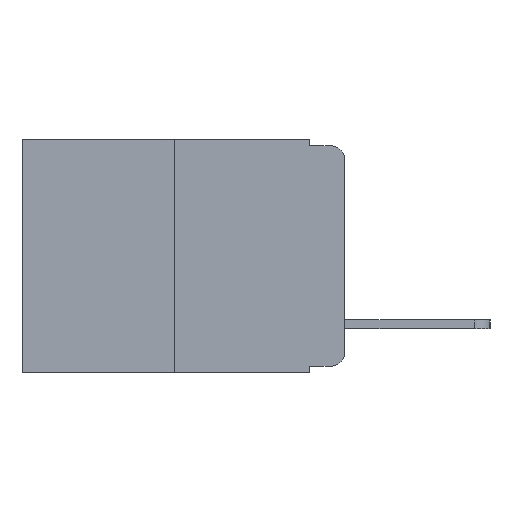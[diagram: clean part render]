
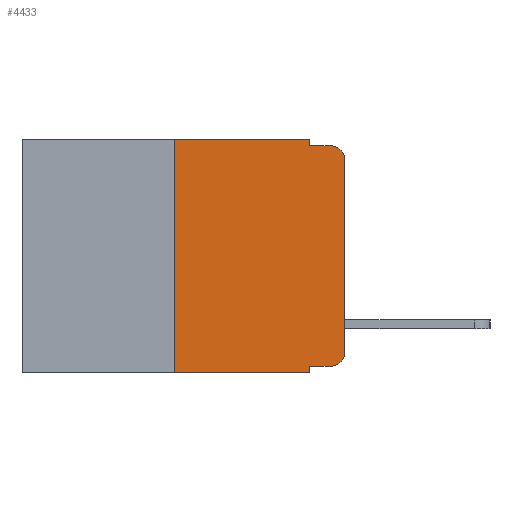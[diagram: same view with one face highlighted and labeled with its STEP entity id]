
A CAD part, left-side view. The second image highlights one B-rep face of the part: STEP entity #4433.
In plain terms, the highlighted planar face has unit normal (-1, 0, 0).
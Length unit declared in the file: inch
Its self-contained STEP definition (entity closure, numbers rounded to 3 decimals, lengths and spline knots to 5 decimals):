
#438 = ORIENTED_EDGE ( 'NONE', *, *, #14048, .F. ) ;
#652 = DIRECTION ( 'NONE',  ( -1., 0., 0. ) ) ;
#881 = EDGE_LOOP ( 'NONE', ( #9283, #4237, #18807, #438, #3809, #8578, #16939, #17595, #15039, #2555 ) ) ;
#1062 = CARTESIAN_POINT ( 'NONE',  ( 0., 0.473, -0.343 ) ) ;
#1090 = CARTESIAN_POINT ( 'NONE',  ( 0., 0.051, -0.01 ) ) ;
#1102 = VERTEX_POINT ( 'NONE', #14629 ) ;
#1168 = CARTESIAN_POINT ( 'NONE',  ( 0., 0.25, -0.343 ) ) ;
#1358 = EDGE_CURVE ( 'NONE', #1861, #6378, #7900, .T. ) ;
#1367 = CARTESIAN_POINT ( 'NONE',  ( 0., 0.473, 0. ) ) ;
#1861 = VERTEX_POINT ( 'NONE', #2861 ) ;
#2159 = DIRECTION ( 'NONE',  ( 0., -1., 0. ) ) ;
#2243 = CARTESIAN_POINT ( 'NONE',  ( 0., 0.473, 0. ) ) ;
#2555 = ORIENTED_EDGE ( 'NONE', *, *, #5660, .T. ) ;
#2861 = CARTESIAN_POINT ( 'NONE',  ( 0., 0.051, -0.333 ) ) ;
#2931 = DIRECTION ( 'NONE',  ( 0., -1., 0. ) ) ;
#2974 = VERTEX_POINT ( 'NONE', #1090 ) ;
#3056 = CARTESIAN_POINT ( 'NONE',  ( 0., 0.02, -0.333 ) ) ;
#3528 = AXIS2_PLACEMENT_3D ( 'NONE', #1367, #14893, #6210 ) ;
#3658 = VECTOR ( 'NONE', #11323, 39.37008 ) ;
#3809 = ORIENTED_EDGE ( 'NONE', *, *, #9143, .F. ) ;
#4237 = ORIENTED_EDGE ( 'NONE', *, *, #10821, .T. ) ;
#4346 = VERTEX_POINT ( 'NONE', #1168 ) ;
#4433 = ADVANCED_FACE ( 'NONE', ( #18304 ), #19179, .F. ) ;
#4644 = DIRECTION ( 'NONE',  ( 0., 0., -1. ) ) ;
#5357 = VERTEX_POINT ( 'NONE', #9347 ) ;
#5660 = EDGE_CURVE ( 'NONE', #6378, #12964, #19162, .T. ) ;
#6019 = CARTESIAN_POINT ( 'NONE',  ( 0., 0.051, -0.333 ) ) ;
#6210 = DIRECTION ( 'NONE',  ( 0., 0., -1. ) ) ;
#6242 = CARTESIAN_POINT ( 'NONE',  ( 0., 0.051, 0. ) ) ;
#6243 = EDGE_CURVE ( 'NONE', #4346, #5357, #9025, .T. ) ;
#6327 = EDGE_CURVE ( 'NONE', #1861, #5357, #8123, .T. ) ;
#6378 = VERTEX_POINT ( 'NONE', #3056 ) ;
#7099 = LINE ( 'NONE', #13309, #15667 ) ;
#7199 = DIRECTION ( 'NONE',  ( -1., 0., 0. ) ) ;
#7653 = CARTESIAN_POINT ( 'NONE',  ( 0., 0.25, 0. ) ) ;
#7676 = VECTOR ( 'NONE', #11834, 39.37008 ) ;
#7782 = LINE ( 'NONE', #8514, #3658 ) ;
#7900 = LINE ( 'NONE', #6019, #11647 ) ;
#8123 = LINE ( 'NONE', #11756, #7676 ) ;
#8327 = CARTESIAN_POINT ( 'NONE',  ( 0., 0., 0. ) ) ;
#8392 = AXIS2_PLACEMENT_3D ( 'NONE', #9902, #652, #11275 ) ;
#8456 = VECTOR ( 'NONE', #9767, 39.37008 ) ;
#8514 = CARTESIAN_POINT ( 'NONE',  ( 0., 0.25, 0. ) ) ;
#8578 = ORIENTED_EDGE ( 'NONE', *, *, #11490, .F. ) ;
#9025 = LINE ( 'NONE', #1062, #17591 ) ;
#9143 = EDGE_CURVE ( 'NONE', #13081, #1102, #17570, .T. ) ;
#9265 = CARTESIAN_POINT ( 'NONE',  ( 0., 0.02, -0.01 ) ) ;
#9283 = ORIENTED_EDGE ( 'NONE', *, *, #13417, .T. ) ;
#9347 = CARTESIAN_POINT ( 'NONE',  ( 0., 0.051, -0.343 ) ) ;
#9767 = DIRECTION ( 'NONE',  ( 0., 0., 1. ) ) ;
#9902 = CARTESIAN_POINT ( 'NONE',  ( 0., 0.02, -0.03 ) ) ;
#10046 = CIRCLE ( 'NONE', #8392, 0.02 ) ;
#10821 = EDGE_CURVE ( 'NONE', #15759, #13163, #10046, .T. ) ;
#11275 = DIRECTION ( 'NONE',  ( 0., 0., -1. ) ) ;
#11323 = DIRECTION ( 'NONE',  ( 0., 0., 1. ) ) ;
#11490 = EDGE_CURVE ( 'NONE', #4346, #13081, #7782, .T. ) ;
#11647 = VECTOR ( 'NONE', #14704, 39.37008 ) ;
#11756 = CARTESIAN_POINT ( 'NONE',  ( 0., 0.051, 0. ) ) ;
#11834 = DIRECTION ( 'NONE',  ( 0., 0., -1. ) ) ;
#11842 = CARTESIAN_POINT ( 'NONE',  ( 0., 0., -0.03 ) ) ;
#12669 = LINE ( 'NONE', #8327, #8456 ) ;
#12964 = VERTEX_POINT ( 'NONE', #17411 ) ;
#13078 = EDGE_CURVE ( 'NONE', #2974, #13163, #7099, .T. ) ;
#13081 = VERTEX_POINT ( 'NONE', #7653 ) ;
#13163 = VERTEX_POINT ( 'NONE', #9265 ) ;
#13219 = VECTOR ( 'NONE', #2159, 39.37008 ) ;
#13309 = CARTESIAN_POINT ( 'NONE',  ( 0., 0.051, -0.01 ) ) ;
#13320 = LINE ( 'NONE', #6242, #17674 ) ;
#13417 = EDGE_CURVE ( 'NONE', #12964, #15759, #12669, .T. ) ;
#14048 = EDGE_CURVE ( 'NONE', #1102, #2974, #13320, .T. ) ;
#14629 = CARTESIAN_POINT ( 'NONE',  ( 0., 0.051, 0. ) ) ;
#14704 = DIRECTION ( 'NONE',  ( 0., -1., 0. ) ) ;
#14893 = DIRECTION ( 'NONE',  ( 1., 0., 0. ) ) ;
#15039 = ORIENTED_EDGE ( 'NONE', *, *, #1358, .T. ) ;
#15667 = VECTOR ( 'NONE', #2931, 39.37008 ) ;
#15759 = VERTEX_POINT ( 'NONE', #11842 ) ;
#15821 = CARTESIAN_POINT ( 'NONE',  ( 0., 0.02, -0.313 ) ) ;
#16053 = DIRECTION ( 'NONE',  ( 0., -1., 0. ) ) ;
#16939 = ORIENTED_EDGE ( 'NONE', *, *, #6243, .T. ) ;
#17288 = DIRECTION ( 'NONE',  ( 0., 0., -1. ) ) ;
#17411 = CARTESIAN_POINT ( 'NONE',  ( 0., 0., -0.313 ) ) ;
#17570 = LINE ( 'NONE', #2243, #13219 ) ;
#17591 = VECTOR ( 'NONE', #16053, 39.37008 ) ;
#17595 = ORIENTED_EDGE ( 'NONE', *, *, #6327, .F. ) ;
#17674 = VECTOR ( 'NONE', #4644, 39.37008 ) ;
#18079 = AXIS2_PLACEMENT_3D ( 'NONE', #15821, #7199, #17288 ) ;
#18304 = FACE_OUTER_BOUND ( 'NONE', #881, .T. ) ;
#18807 = ORIENTED_EDGE ( 'NONE', *, *, #13078, .F. ) ;
#19162 = CIRCLE ( 'NONE', #18079, 0.02 ) ;
#19179 = PLANE ( 'NONE',  #3528 ) ;
